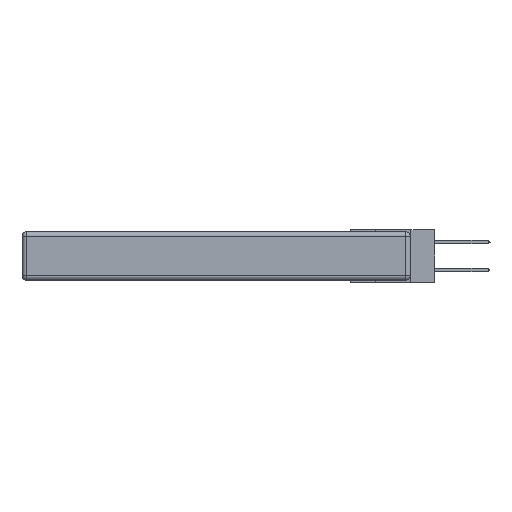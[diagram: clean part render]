
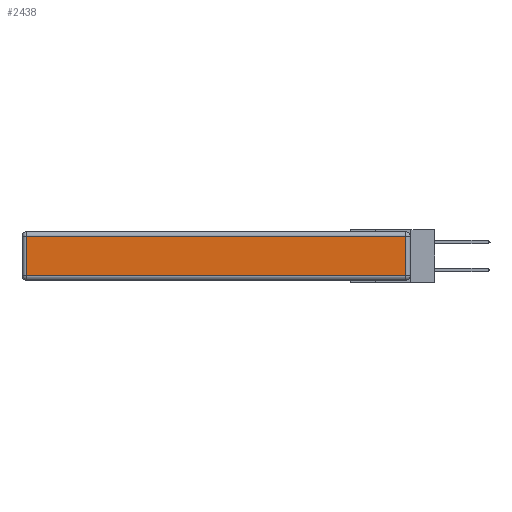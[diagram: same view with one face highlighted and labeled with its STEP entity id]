
A CAD part, left-side view. The second image highlights one B-rep face of the part: STEP entity #2438.
In plain terms, the highlighted planar face has unit normal (-1, 0, 0).
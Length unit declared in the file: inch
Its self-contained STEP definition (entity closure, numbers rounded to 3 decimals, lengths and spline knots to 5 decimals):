
#1113 = CARTESIAN_POINT ( 'NONE',  ( 0., 0., -0.343 ) ) ;
#1125 = CARTESIAN_POINT ( 'NONE',  ( 0., 0.03, -0.313 ) ) ;
#1249 = LINE ( 'NONE', #13015, #21312 ) ;
#2438 = ADVANCED_FACE ( 'NONE', ( #16771 ), #11698, .T. ) ;
#2589 = LINE ( 'NONE', #20800, #27355 ) ;
#3810 = CARTESIAN_POINT ( 'NONE',  ( 0., 0.03, -0.03 ) ) ;
#4796 = EDGE_CURVE ( 'NONE', #24482, #18227, #19310, .T. ) ;
#6316 = VECTOR ( 'NONE', #20886, 39.37008 ) ;
#6544 = EDGE_CURVE ( 'NONE', #8376, #24482, #22774, .T. ) ;
#7093 = VECTOR ( 'NONE', #13200, 39.37008 ) ;
#8376 = VERTEX_POINT ( 'NONE', #3810 ) ;
#9197 = ORIENTED_EDGE ( 'NONE', *, *, #15941, .T. ) ;
#9721 = DIRECTION ( 'NONE',  ( -1., 0., 0. ) ) ;
#10093 = EDGE_LOOP ( 'NONE', ( #10111, #9197, #21782, #12188 ) ) ;
#10111 = ORIENTED_EDGE ( 'NONE', *, *, #15536, .T. ) ;
#11698 = PLANE ( 'NONE',  #15446 ) ;
#12188 = ORIENTED_EDGE ( 'NONE', *, *, #4796, .T. ) ;
#12223 = VERTEX_POINT ( 'NONE', #1125 ) ;
#12398 = CARTESIAN_POINT ( 'NONE',  ( 0., 2.72, -0.343 ) ) ;
#13015 = CARTESIAN_POINT ( 'NONE',  ( 0., 0., -0.313 ) ) ;
#13200 = DIRECTION ( 'NONE',  ( 0., 1., 0. ) ) ;
#13922 = DIRECTION ( 'NONE',  ( 0., 0., 1. ) ) ;
#14846 = DIRECTION ( 'NONE',  ( 0., -1., 0. ) ) ;
#15446 = AXIS2_PLACEMENT_3D ( 'NONE', #1113, #9721, #13922 ) ;
#15536 = EDGE_CURVE ( 'NONE', #18227, #12223, #1249, .T. ) ;
#15941 = EDGE_CURVE ( 'NONE', #12223, #8376, #2589, .T. ) ;
#16493 = DIRECTION ( 'NONE',  ( 0., 0., 1. ) ) ;
#16771 = FACE_OUTER_BOUND ( 'NONE', #10093, .T. ) ;
#18227 = VERTEX_POINT ( 'NONE', #19918 ) ;
#19237 = CARTESIAN_POINT ( 'NONE',  ( 0., 2.72, -0.03 ) ) ;
#19310 = LINE ( 'NONE', #12398, #6316 ) ;
#19918 = CARTESIAN_POINT ( 'NONE',  ( 0., 2.72, -0.313 ) ) ;
#20800 = CARTESIAN_POINT ( 'NONE',  ( 0., 0.03, -0.343 ) ) ;
#20886 = DIRECTION ( 'NONE',  ( 0., 0., -1. ) ) ;
#21312 = VECTOR ( 'NONE', #14846, 39.37008 ) ;
#21782 = ORIENTED_EDGE ( 'NONE', *, *, #6544, .T. ) ;
#22774 = LINE ( 'NONE', #24011, #7093 ) ;
#24011 = CARTESIAN_POINT ( 'NONE',  ( 0., 2.75, -0.03 ) ) ;
#24482 = VERTEX_POINT ( 'NONE', #19237 ) ;
#27355 = VECTOR ( 'NONE', #16493, 39.37008 ) ;
